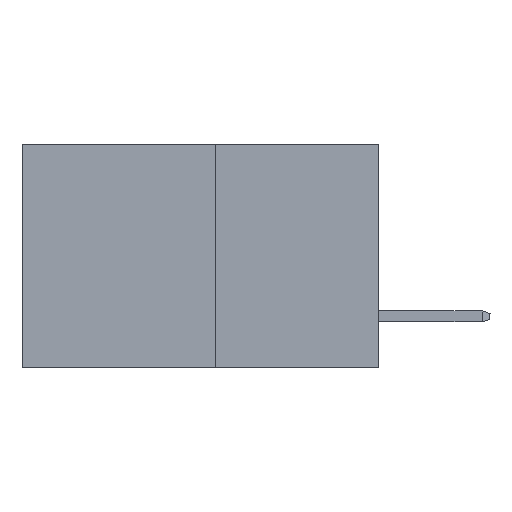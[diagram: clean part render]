
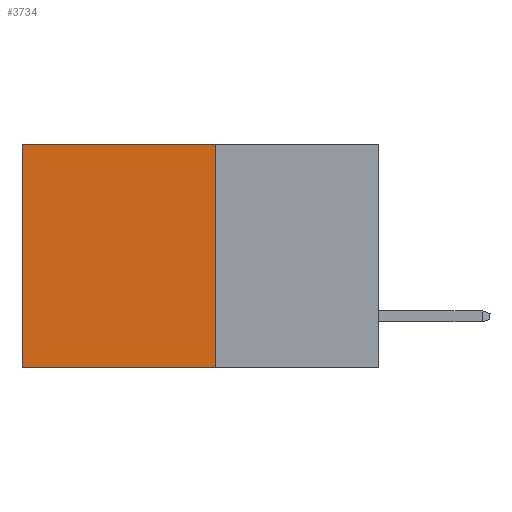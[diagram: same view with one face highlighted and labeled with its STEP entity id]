
A CAD part, left-side view. The second image highlights one B-rep face of the part: STEP entity #3734.
In plain terms, the highlighted planar face has unit normal (-1, 0, 0).
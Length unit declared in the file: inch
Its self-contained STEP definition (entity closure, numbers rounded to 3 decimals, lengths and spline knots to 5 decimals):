
#377 = DIRECTION ( 'NONE',  ( 0., 0., -1. ) ) ;
#1738 = ORIENTED_EDGE ( 'NONE', *, *, #25167, .F. ) ;
#2021 = CARTESIAN_POINT ( 'NONE',  ( 0.277, 0.27, -0.37 ) ) ;
#3734 = ADVANCED_FACE ( 'NONE', ( #9594 ), #10246, .F. ) ;
#5234 = CARTESIAN_POINT ( 'NONE',  ( 0.277, 0.27, -0.37 ) ) ;
#6303 = VECTOR ( 'NONE', #9741, 39.37008 ) ;
#7559 = DIRECTION ( 'NONE',  ( 0., 0., -1. ) ) ;
#7661 = VERTEX_POINT ( 'NONE', #16220 ) ;
#8925 = DIRECTION ( 'NONE',  ( 0., 1., 0. ) ) ;
#9110 = ORIENTED_EDGE ( 'NONE', *, *, #27685, .F. ) ;
#9594 = FACE_OUTER_BOUND ( 'NONE', #10269, .T. ) ;
#9741 = DIRECTION ( 'NONE',  ( 0., 1., 0. ) ) ;
#10200 = LINE ( 'NONE', #5234, #21862 ) ;
#10246 = PLANE ( 'NONE',  #28516 ) ;
#10269 = EDGE_LOOP ( 'NONE', ( #16960, #1738, #9110, #12014 ) ) ;
#10416 = LINE ( 'NONE', #28229, #15173 ) ;
#10516 = CARTESIAN_POINT ( 'NONE',  ( 0.277, 0.59, -0.37 ) ) ;
#10636 = VERTEX_POINT ( 'NONE', #20356 ) ;
#10934 = EDGE_CURVE ( 'NONE', #10636, #7661, #18651, .T. ) ;
#11171 = VERTEX_POINT ( 'NONE', #10516 ) ;
#12014 = ORIENTED_EDGE ( 'NONE', *, *, #10934, .T. ) ;
#12184 = VECTOR ( 'NONE', #8925, 39.37008 ) ;
#12579 = CARTESIAN_POINT ( 'NONE',  ( 0.277, 0.27, -0.37 ) ) ;
#14933 = DIRECTION ( 'NONE',  ( 0., 0., -1. ) ) ;
#15173 = VECTOR ( 'NONE', #377, 39.37008 ) ;
#16220 = CARTESIAN_POINT ( 'NONE',  ( 0.277, 0.59, 0. ) ) ;
#16960 = ORIENTED_EDGE ( 'NONE', *, *, #29476, .T. ) ;
#18651 = LINE ( 'NONE', #21363, #6303 ) ;
#20356 = CARTESIAN_POINT ( 'NONE',  ( 0.277, 0.27, 0. ) ) ;
#21363 = CARTESIAN_POINT ( 'NONE',  ( 0.277, 0.27, 0. ) ) ;
#21862 = VECTOR ( 'NONE', #7559, 39.37008 ) ;
#25167 = EDGE_CURVE ( 'NONE', #25957, #11171, #30014, .T. ) ;
#25957 = VERTEX_POINT ( 'NONE', #27808 ) ;
#27685 = EDGE_CURVE ( 'NONE', #10636, #25957, #10200, .T. ) ;
#27808 = CARTESIAN_POINT ( 'NONE',  ( 0.277, 0.27, -0.37 ) ) ;
#28229 = CARTESIAN_POINT ( 'NONE',  ( 0.277, 0.59, -0.37 ) ) ;
#28516 = AXIS2_PLACEMENT_3D ( 'NONE', #12579, #28839, #14933 ) ;
#28839 = DIRECTION ( 'NONE',  ( 1., 0., 0. ) ) ;
#29476 = EDGE_CURVE ( 'NONE', #7661, #11171, #10416, .T. ) ;
#30014 = LINE ( 'NONE', #2021, #12184 ) ;
